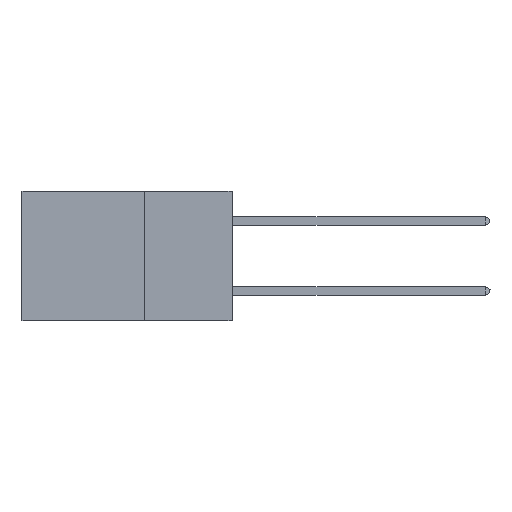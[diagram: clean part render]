
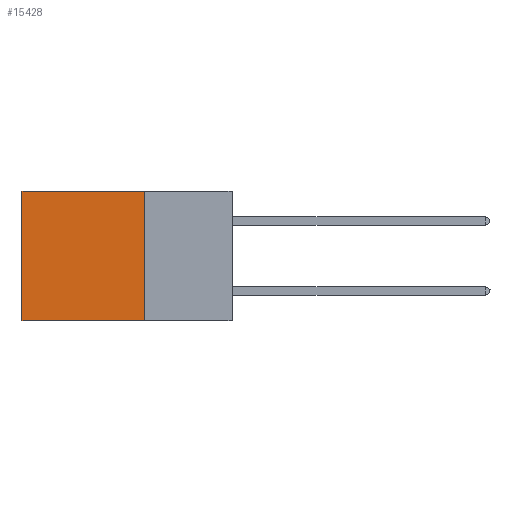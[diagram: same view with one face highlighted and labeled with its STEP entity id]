
A CAD part, left-side view. The second image highlights one B-rep face of the part: STEP entity #15428.
In plain terms, the highlighted planar face has unit normal (-1, 0, 0).
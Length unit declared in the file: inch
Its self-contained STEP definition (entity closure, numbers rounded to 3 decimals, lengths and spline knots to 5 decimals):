
#344 = CARTESIAN_POINT ( 'NONE',  ( 0.2875, 0.25, 0. ) ) ;
#463 = EDGE_CURVE ( 'NONE', #16413, #6024, #8761, .T. ) ;
#707 = ORIENTED_EDGE ( 'NONE', *, *, #15434, .F. ) ;
#1248 = DIRECTION ( 'NONE',  ( 0., 0., -1. ) ) ;
#1880 = DIRECTION ( 'NONE',  ( 0., 0., -1. ) ) ;
#3361 = ORIENTED_EDGE ( 'NONE', *, *, #3799, .T. ) ;
#3659 = VECTOR ( 'NONE', #22001, 39.37008 ) ;
#3720 = CARTESIAN_POINT ( 'NONE',  ( 0.2875, 0.25, -0.37 ) ) ;
#3799 = EDGE_CURVE ( 'NONE', #16413, #14999, #20036, .T. ) ;
#4013 = ORIENTED_EDGE ( 'NONE', *, *, #463, .F. ) ;
#4424 = VECTOR ( 'NONE', #1248, 39.37008 ) ;
#4778 = FACE_OUTER_BOUND ( 'NONE', #13353, .T. ) ;
#5611 = PLANE ( 'NONE',  #16595 ) ;
#6024 = VERTEX_POINT ( 'NONE', #13285 ) ;
#8725 = VECTOR ( 'NONE', #21259, 39.37008 ) ;
#8761 = LINE ( 'NONE', #10634, #4424 ) ;
#9067 = CARTESIAN_POINT ( 'NONE',  ( 0.2875, 0.6, 0. ) ) ;
#10605 = CARTESIAN_POINT ( 'NONE',  ( 0.2875, 0.6, 0. ) ) ;
#10634 = CARTESIAN_POINT ( 'NONE',  ( 0.2875, 0.25, 0. ) ) ;
#11188 = CARTESIAN_POINT ( 'NONE',  ( 0.2875, 0.25, 0. ) ) ;
#11391 = CARTESIAN_POINT ( 'NONE',  ( 0.2875, 0.6, -0.37 ) ) ;
#13285 = CARTESIAN_POINT ( 'NONE',  ( 0.2875, 0.25, -0.37 ) ) ;
#13353 = EDGE_LOOP ( 'NONE', ( #17760, #707, #4013, #3361 ) ) ;
#13370 = CARTESIAN_POINT ( 'NONE',  ( 0.2875, 0.25, 0. ) ) ;
#14999 = VERTEX_POINT ( 'NONE', #9067 ) ;
#15061 = VERTEX_POINT ( 'NONE', #11391 ) ;
#15428 = ADVANCED_FACE ( 'NONE', ( #4778 ), #5611, .F. ) ;
#15434 = EDGE_CURVE ( 'NONE', #6024, #15061, #23725, .T. ) ;
#16033 = VECTOR ( 'NONE', #18863, 39.37008 ) ;
#16413 = VERTEX_POINT ( 'NONE', #13370 ) ;
#16595 = AXIS2_PLACEMENT_3D ( 'NONE', #11188, #20450, #1880 ) ;
#17760 = ORIENTED_EDGE ( 'NONE', *, *, #23402, .T. ) ;
#18863 = DIRECTION ( 'NONE',  ( 0., 1., 0. ) ) ;
#19349 = LINE ( 'NONE', #10605, #8725 ) ;
#20036 = LINE ( 'NONE', #344, #16033 ) ;
#20450 = DIRECTION ( 'NONE',  ( 1., 0., 0. ) ) ;
#21259 = DIRECTION ( 'NONE',  ( 0., 0., -1. ) ) ;
#22001 = DIRECTION ( 'NONE',  ( 0., 1., 0. ) ) ;
#23402 = EDGE_CURVE ( 'NONE', #14999, #15061, #19349, .T. ) ;
#23725 = LINE ( 'NONE', #3720, #3659 ) ;
